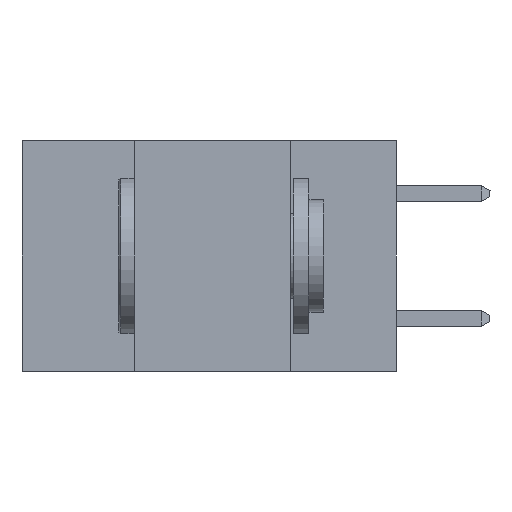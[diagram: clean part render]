
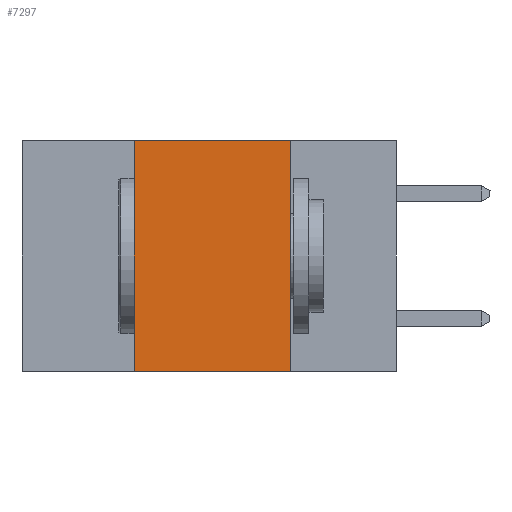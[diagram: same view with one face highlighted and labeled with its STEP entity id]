
A CAD part, left-side view. The second image highlights one B-rep face of the part: STEP entity #7297.
In plain terms, the highlighted planar face has unit normal (-1, 0, 0).
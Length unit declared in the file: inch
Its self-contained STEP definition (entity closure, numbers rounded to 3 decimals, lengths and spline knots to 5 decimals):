
#1347 = EDGE_CURVE ( 'NONE', #12292, #6124, #12623, .T. ) ;
#1731 = DIRECTION ( 'NONE',  ( 0., -1., 0. ) ) ;
#2692 = VECTOR ( 'NONE', #7350, 39.37008 ) ;
#3011 = CARTESIAN_POINT ( 'NONE',  ( 0., 0.6, 0. ) ) ;
#3109 = AXIS2_PLACEMENT_3D ( 'NONE', #3729, #10927, #4777 ) ;
#3696 = EDGE_CURVE ( 'NONE', #5173, #9513, #6933, .T. ) ;
#3729 = CARTESIAN_POINT ( 'NONE',  ( 0., 0.6, 0. ) ) ;
#3769 = CARTESIAN_POINT ( 'NONE',  ( 0., 0.17, 0. ) ) ;
#4184 = CARTESIAN_POINT ( 'NONE',  ( 0., 0.6, -0.37 ) ) ;
#4777 = DIRECTION ( 'NONE',  ( 0., 0., -1. ) ) ;
#5173 = VERTEX_POINT ( 'NONE', #7174 ) ;
#5248 = EDGE_CURVE ( 'NONE', #5173, #6124, #11306, .T. ) ;
#5806 = LINE ( 'NONE', #3011, #8264 ) ;
#5994 = DIRECTION ( 'NONE',  ( 0., 0., -1. ) ) ;
#6124 = VERTEX_POINT ( 'NONE', #6309 ) ;
#6309 = CARTESIAN_POINT ( 'NONE',  ( 0., 0.17, -0.37 ) ) ;
#6932 = ORIENTED_EDGE ( 'NONE', *, *, #1347, .F. ) ;
#6933 = LINE ( 'NONE', #10823, #12698 ) ;
#7169 = ORIENTED_EDGE ( 'NONE', *, *, #5248, .T. ) ;
#7174 = CARTESIAN_POINT ( 'NONE',  ( 0., 0.42, -0.37 ) ) ;
#7177 = VECTOR ( 'NONE', #5994, 39.37008 ) ;
#7297 = ADVANCED_FACE ( 'NONE', ( #13260 ), #9925, .F. ) ;
#7350 = DIRECTION ( 'NONE',  ( 0., -1., 0. ) ) ;
#7666 = EDGE_CURVE ( 'NONE', #9513, #12292, #5806, .T. ) ;
#8264 = VECTOR ( 'NONE', #1731, 39.37008 ) ;
#8725 = CARTESIAN_POINT ( 'NONE',  ( 0., 0.17, 0. ) ) ;
#9513 = VERTEX_POINT ( 'NONE', #11304 ) ;
#9538 = DIRECTION ( 'NONE',  ( 0., 0., 1. ) ) ;
#9925 = PLANE ( 'NONE',  #3109 ) ;
#10823 = CARTESIAN_POINT ( 'NONE',  ( 0., 0.42, 0. ) ) ;
#10927 = DIRECTION ( 'NONE',  ( 1., 0., 0. ) ) ;
#11094 = EDGE_LOOP ( 'NONE', ( #6932, #11806, #11234, #7169 ) ) ;
#11234 = ORIENTED_EDGE ( 'NONE', *, *, #3696, .F. ) ;
#11304 = CARTESIAN_POINT ( 'NONE',  ( 0., 0.42, 0. ) ) ;
#11306 = LINE ( 'NONE', #4184, #2692 ) ;
#11806 = ORIENTED_EDGE ( 'NONE', *, *, #7666, .F. ) ;
#12292 = VERTEX_POINT ( 'NONE', #3769 ) ;
#12623 = LINE ( 'NONE', #8725, #7177 ) ;
#12698 = VECTOR ( 'NONE', #9538, 39.37008 ) ;
#13260 = FACE_OUTER_BOUND ( 'NONE', #11094, .T. ) ;
